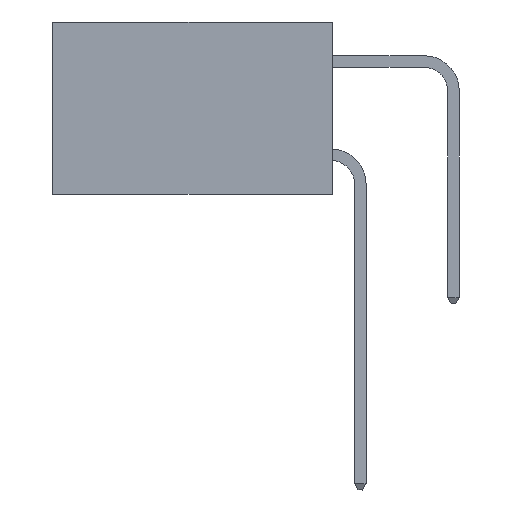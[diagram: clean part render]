
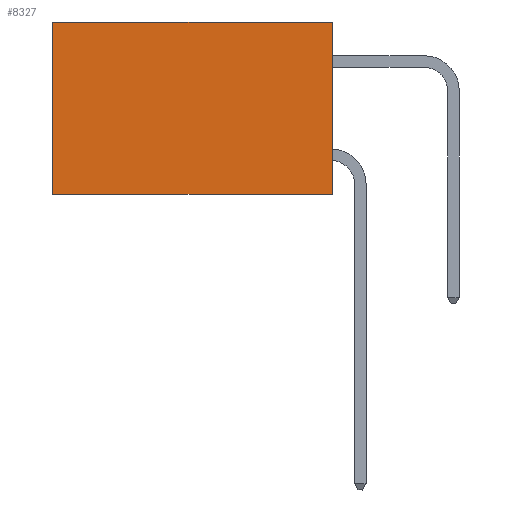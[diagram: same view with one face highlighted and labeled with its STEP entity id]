
A CAD part, left-side view. The second image highlights one B-rep face of the part: STEP entity #8327.
In plain terms, the highlighted planar face has unit normal (-1, 0, 0).
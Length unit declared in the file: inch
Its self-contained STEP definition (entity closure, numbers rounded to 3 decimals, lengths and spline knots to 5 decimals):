
#112 = CARTESIAN_POINT ( 'NONE',  ( 0.298, 0.6, -0.37 ) ) ;
#178 = EDGE_LOOP ( 'NONE', ( #6381, #7164, #1883, #3676 ) ) ;
#736 = CARTESIAN_POINT ( 'NONE',  ( 0.298, 0.6, 0. ) ) ;
#1384 = CARTESIAN_POINT ( 'NONE',  ( 0.298, 0., 0. ) ) ;
#1547 = VECTOR ( 'NONE', #7316, 39.37008 ) ;
#1858 = LINE ( 'NONE', #1384, #9105 ) ;
#1883 = ORIENTED_EDGE ( 'NONE', *, *, #7045, .F. ) ;
#2008 = PLANE ( 'NONE',  #8608 ) ;
#2396 = LINE ( 'NONE', #5421, #1547 ) ;
#2419 = VERTEX_POINT ( 'NONE', #6960 ) ;
#2766 = DIRECTION ( 'NONE',  ( 1., 0., 0. ) ) ;
#3676 = ORIENTED_EDGE ( 'NONE', *, *, #8621, .T. ) ;
#3960 = EDGE_CURVE ( 'NONE', #6727, #5454, #11091, .T. ) ;
#4502 = CARTESIAN_POINT ( 'NONE',  ( 0.298, 0., 0. ) ) ;
#5136 = DIRECTION ( 'NONE',  ( 0., 0., -1. ) ) ;
#5381 = DIRECTION ( 'NONE',  ( 0., 0., -1. ) ) ;
#5421 = CARTESIAN_POINT ( 'NONE',  ( 0.298, 0., 0. ) ) ;
#5454 = VERTEX_POINT ( 'NONE', #112 ) ;
#5490 = VECTOR ( 'NONE', #7982, 39.37008 ) ;
#6381 = ORIENTED_EDGE ( 'NONE', *, *, #9737, .T. ) ;
#6727 = VERTEX_POINT ( 'NONE', #9492 ) ;
#6879 = CARTESIAN_POINT ( 'NONE',  ( 0.298, 0., 0. ) ) ;
#6960 = CARTESIAN_POINT ( 'NONE',  ( 0.298, 0.6, 0. ) ) ;
#7045 = EDGE_CURVE ( 'NONE', #7621, #6727, #1858, .T. ) ;
#7164 = ORIENTED_EDGE ( 'NONE', *, *, #3960, .F. ) ;
#7316 = DIRECTION ( 'NONE',  ( 0., 1., 0. ) ) ;
#7621 = VERTEX_POINT ( 'NONE', #6879 ) ;
#7982 = DIRECTION ( 'NONE',  ( 0., 1., 0. ) ) ;
#8085 = FACE_OUTER_BOUND ( 'NONE', #178, .T. ) ;
#8327 = ADVANCED_FACE ( 'NONE', ( #8085 ), #2008, .F. ) ;
#8608 = AXIS2_PLACEMENT_3D ( 'NONE', #4502, #2766, #5381 ) ;
#8621 = EDGE_CURVE ( 'NONE', #7621, #2419, #2396, .T. ) ;
#8866 = CARTESIAN_POINT ( 'NONE',  ( 0.298, 0., -0.37 ) ) ;
#9105 = VECTOR ( 'NONE', #11151, 39.37008 ) ;
#9492 = CARTESIAN_POINT ( 'NONE',  ( 0.298, 0., -0.37 ) ) ;
#9670 = LINE ( 'NONE', #736, #9939 ) ;
#9737 = EDGE_CURVE ( 'NONE', #2419, #5454, #9670, .T. ) ;
#9939 = VECTOR ( 'NONE', #5136, 39.37008 ) ;
#11091 = LINE ( 'NONE', #8866, #5490 ) ;
#11151 = DIRECTION ( 'NONE',  ( 0., 0., -1. ) ) ;
